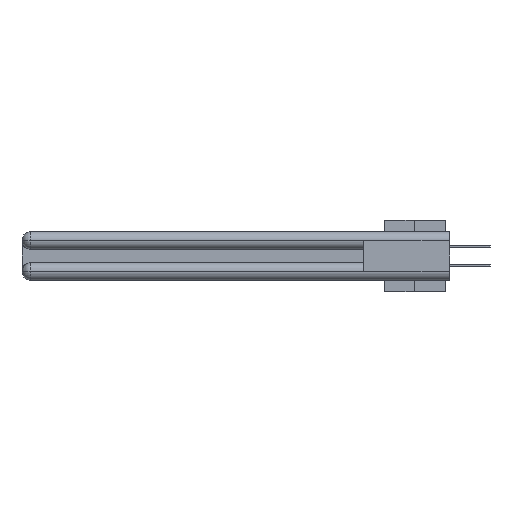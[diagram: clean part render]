
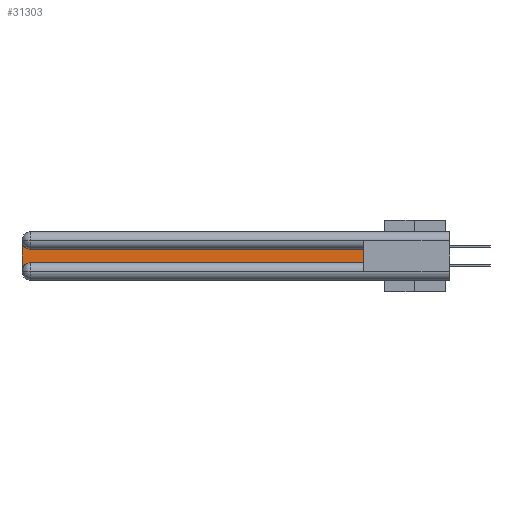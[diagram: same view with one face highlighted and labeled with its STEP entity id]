
A CAD part, left-side view. The second image highlights one B-rep face of the part: STEP entity #31303.
In plain terms, the highlighted planar face has unit normal (-1, 0, 0).
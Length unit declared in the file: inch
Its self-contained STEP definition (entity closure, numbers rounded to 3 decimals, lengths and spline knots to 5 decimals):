
#1839 = DIRECTION ( 'NONE',  ( 0., 0., 1. ) ) ;
#2475 = AXIS2_PLACEMENT_3D ( 'NONE', #14606, #35578, #26773 ) ;
#3514 = CARTESIAN_POINT ( 'NONE',  ( 0.075, 0.6, -0.2175 ) ) ;
#3930 = VECTOR ( 'NONE', #1839, 39.37008 ) ;
#5057 = DIRECTION ( 'NONE',  ( 0., 0., -1. ) ) ;
#6051 = CARTESIAN_POINT ( 'NONE',  ( 0.075, 3., -0.1225 ) ) ;
#6199 = DIRECTION ( 'NONE',  ( 0., 0., -1. ) ) ;
#6350 = CARTESIAN_POINT ( 'NONE',  ( 0.075, 3., -0.0625 ) ) ;
#9166 = EDGE_LOOP ( 'NONE', ( #14283, #16998, #9923, #37171, #13817, #26563 ) ) ;
#9459 = CARTESIAN_POINT ( 'NONE',  ( 0.075, 2.94, -0.1225 ) ) ;
#9923 = ORIENTED_EDGE ( 'NONE', *, *, #18892, .T. ) ;
#13085 = CARTESIAN_POINT ( 'NONE',  ( 0.075, 3., -0.2775 ) ) ;
#13519 = VECTOR ( 'NONE', #6199, 39.37008 ) ;
#13817 = ORIENTED_EDGE ( 'NONE', *, *, #22092, .T. ) ;
#14025 = CARTESIAN_POINT ( 'NONE',  ( 0.075, 2.94, -0.0625 ) ) ;
#14283 = ORIENTED_EDGE ( 'NONE', *, *, #24759, .T. ) ;
#14606 = CARTESIAN_POINT ( 'NONE',  ( 0.075, 2.94, -0.2775 ) ) ;
#14900 = VERTEX_POINT ( 'NONE', #13085 ) ;
#16998 = ORIENTED_EDGE ( 'NONE', *, *, #23954, .T. ) ;
#17686 = DIRECTION ( 'NONE',  ( 0., -1., 0. ) ) ;
#17826 = VERTEX_POINT ( 'NONE', #36778 ) ;
#18556 = FACE_OUTER_BOUND ( 'NONE', #9166, .T. ) ;
#18892 = EDGE_CURVE ( 'NONE', #28813, #14900, #19552, .T. ) ;
#19552 = LINE ( 'NONE', #35355, #13519 ) ;
#20132 = CARTESIAN_POINT ( 'NONE',  ( 0.075, 0.6, -0.1225 ) ) ;
#20178 = CARTESIAN_POINT ( 'NONE',  ( 0.075, 0.6, -0.2175 ) ) ;
#20814 = VECTOR ( 'NONE', #26589, 39.37008 ) ;
#21710 = LINE ( 'NONE', #32108, #20814 ) ;
#21994 = LINE ( 'NONE', #34490, #3930 ) ;
#22092 = EDGE_CURVE ( 'NONE', #17826, #23689, #31898, .T. ) ;
#22536 = VECTOR ( 'NONE', #17686, 39.37008 ) ;
#23689 = VERTEX_POINT ( 'NONE', #3514 ) ;
#23786 = PLANE ( 'NONE',  #25942 ) ;
#23954 = EDGE_CURVE ( 'NONE', #30398, #28813, #38127, .T. ) ;
#24759 = EDGE_CURVE ( 'NONE', #36800, #30398, #21710, .T. ) ;
#25942 = AXIS2_PLACEMENT_3D ( 'NONE', #6051, #38440, #32432 ) ;
#26563 = ORIENTED_EDGE ( 'NONE', *, *, #35018, .T. ) ;
#26589 = DIRECTION ( 'NONE',  ( 0., 1., 0. ) ) ;
#26773 = DIRECTION ( 'NONE',  ( 0., 0., -1. ) ) ;
#28813 = VERTEX_POINT ( 'NONE', #6350 ) ;
#28830 = CIRCLE ( 'NONE', #2475, 0.06 ) ;
#30398 = VERTEX_POINT ( 'NONE', #9459 ) ;
#31303 = ADVANCED_FACE ( 'NONE', ( #18556 ), #23786, .F. ) ;
#31898 = LINE ( 'NONE', #20178, #22536 ) ;
#32108 = CARTESIAN_POINT ( 'NONE',  ( 0.075, 0.6, -0.1225 ) ) ;
#32432 = DIRECTION ( 'NONE',  ( 0., 0., -1. ) ) ;
#33354 = AXIS2_PLACEMENT_3D ( 'NONE', #14025, #34859, #5057 ) ;
#34490 = CARTESIAN_POINT ( 'NONE',  ( 0.075, 0.6, -0.2175 ) ) ;
#34859 = DIRECTION ( 'NONE',  ( 1., 0., 0. ) ) ;
#35018 = EDGE_CURVE ( 'NONE', #23689, #36800, #21994, .T. ) ;
#35355 = CARTESIAN_POINT ( 'NONE',  ( 0.075, 3., -0.2175 ) ) ;
#35578 = DIRECTION ( 'NONE',  ( 1., 0., 0. ) ) ;
#36778 = CARTESIAN_POINT ( 'NONE',  ( 0.075, 2.94, -0.2175 ) ) ;
#36800 = VERTEX_POINT ( 'NONE', #20132 ) ;
#37171 = ORIENTED_EDGE ( 'NONE', *, *, #37477, .T. ) ;
#37477 = EDGE_CURVE ( 'NONE', #14900, #17826, #28830, .T. ) ;
#38127 = CIRCLE ( 'NONE', #33354, 0.06 ) ;
#38440 = DIRECTION ( 'NONE',  ( 1., 0., 0. ) ) ;
